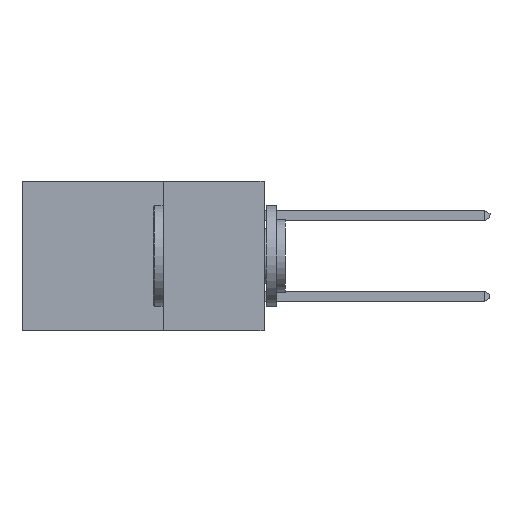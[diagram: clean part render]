
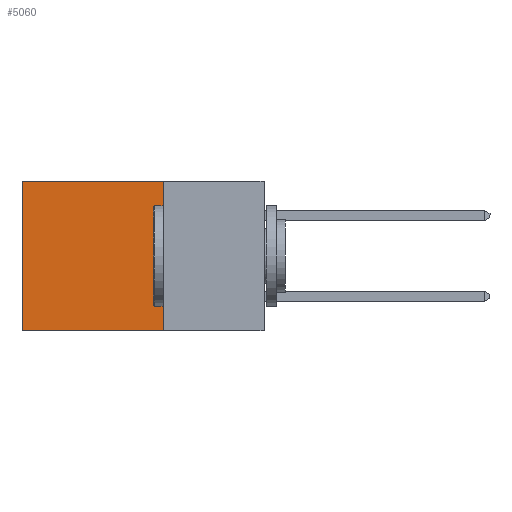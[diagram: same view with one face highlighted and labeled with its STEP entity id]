
A CAD part, left-side view. The second image highlights one B-rep face of the part: STEP entity #5060.
In plain terms, the highlighted planar face has unit normal (-1, 0, 0).
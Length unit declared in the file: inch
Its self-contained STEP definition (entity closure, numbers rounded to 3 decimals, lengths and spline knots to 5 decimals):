
#660 = DIRECTION ( 'NONE',  ( 0., 1., 0. ) ) ;
#3274 = CARTESIAN_POINT ( 'NONE',  ( 0.298, 0.6, -0.37 ) ) ;
#3600 = VERTEX_POINT ( 'NONE', #3954 ) ;
#3954 = CARTESIAN_POINT ( 'NONE',  ( 0.298, 0.25, 0. ) ) ;
#5060 = ADVANCED_FACE ( 'NONE', ( #12332 ), #22890, .F. ) ;
#5604 = DIRECTION ( 'NONE',  ( 0., 0., -1. ) ) ;
#6304 = CARTESIAN_POINT ( 'NONE',  ( 0.298, 0.25, 0. ) ) ;
#6600 = VECTOR ( 'NONE', #660, 39.37008 ) ;
#8569 = EDGE_CURVE ( 'NONE', #3600, #21733, #10041, .T. ) ;
#8604 = VECTOR ( 'NONE', #5604, 39.37008 ) ;
#10041 = LINE ( 'NONE', #10985, #20433 ) ;
#10468 = DIRECTION ( 'NONE',  ( 1., 0., 0. ) ) ;
#10985 = CARTESIAN_POINT ( 'NONE',  ( 0.298, 0.25, 0. ) ) ;
#11268 = VERTEX_POINT ( 'NONE', #3274 ) ;
#11794 = EDGE_CURVE ( 'NONE', #21733, #11268, #17017, .T. ) ;
#12187 = ORIENTED_EDGE ( 'NONE', *, *, #21950, .T. ) ;
#12332 = FACE_OUTER_BOUND ( 'NONE', #16616, .T. ) ;
#13076 = DIRECTION ( 'NONE',  ( 0., 0., -1. ) ) ;
#13162 = VECTOR ( 'NONE', #22585, 39.37008 ) ;
#14013 = CARTESIAN_POINT ( 'NONE',  ( 0.298, 0.6, 0. ) ) ;
#14150 = LINE ( 'NONE', #18000, #8604 ) ;
#16616 = EDGE_LOOP ( 'NONE', ( #22430, #22898, #17769, #12187 ) ) ;
#17017 = LINE ( 'NONE', #23444, #6600 ) ;
#17479 = VERTEX_POINT ( 'NONE', #14013 ) ;
#17769 = ORIENTED_EDGE ( 'NONE', *, *, #8569, .F. ) ;
#17930 = CARTESIAN_POINT ( 'NONE',  ( 0.298, 0.25, -0.37 ) ) ;
#18000 = CARTESIAN_POINT ( 'NONE',  ( 0.298, 0.6, 0. ) ) ;
#18160 = EDGE_CURVE ( 'NONE', #17479, #11268, #14150, .T. ) ;
#20433 = VECTOR ( 'NONE', #13076, 39.37008 ) ;
#21733 = VERTEX_POINT ( 'NONE', #17930 ) ;
#21950 = EDGE_CURVE ( 'NONE', #3600, #17479, #24783, .T. ) ;
#22280 = AXIS2_PLACEMENT_3D ( 'NONE', #6304, #10468, #24940 ) ;
#22430 = ORIENTED_EDGE ( 'NONE', *, *, #18160, .T. ) ;
#22585 = DIRECTION ( 'NONE',  ( 0., 1., 0. ) ) ;
#22890 = PLANE ( 'NONE',  #22280 ) ;
#22898 = ORIENTED_EDGE ( 'NONE', *, *, #11794, .F. ) ;
#23444 = CARTESIAN_POINT ( 'NONE',  ( 0.298, 0.25, -0.37 ) ) ;
#24783 = LINE ( 'NONE', #26573, #13162 ) ;
#24940 = DIRECTION ( 'NONE',  ( 0., 0., -1. ) ) ;
#26573 = CARTESIAN_POINT ( 'NONE',  ( 0.298, 0.25, 0. ) ) ;
